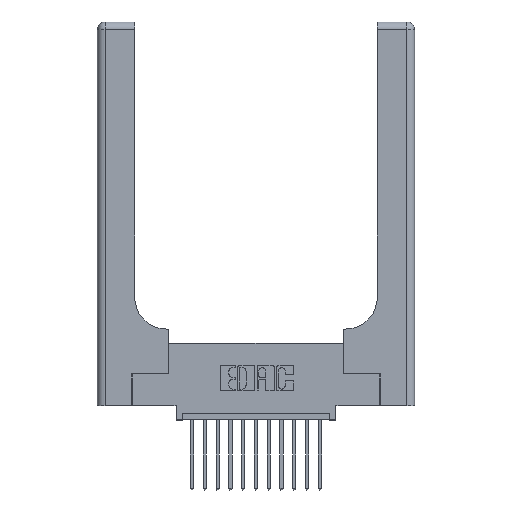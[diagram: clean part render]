
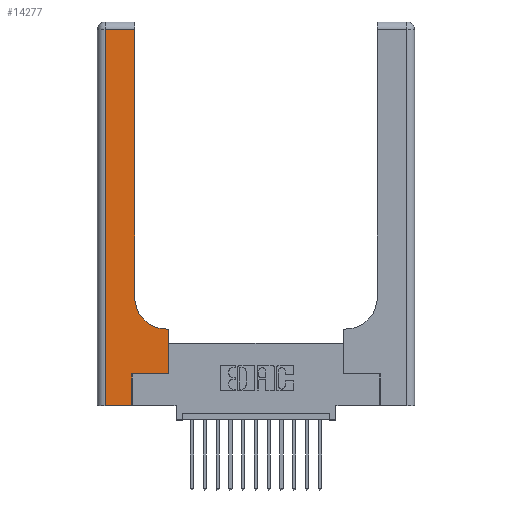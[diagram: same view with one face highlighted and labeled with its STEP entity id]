
A CAD part, top view. The second image highlights one B-rep face of the part: STEP entity #14277.
In plain terms, the highlighted planar face has unit normal (0, 0, 1).
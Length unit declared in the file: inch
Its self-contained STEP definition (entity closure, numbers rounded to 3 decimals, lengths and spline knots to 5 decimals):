
#93 = LINE ( 'NONE', #13680, #14553 ) ;
#414 = EDGE_CURVE ( 'NONE', #13971, #17429, #8022, .T. ) ;
#449 = CARTESIAN_POINT ( 'NONE',  ( 0.269, 0.25, 0.37 ) ) ;
#641 = DIRECTION ( 'NONE',  ( 0., 1., 0. ) ) ;
#719 = DIRECTION ( 'NONE',  ( -1., 0., 0. ) ) ;
#744 = VECTOR ( 'NONE', #3154, 39.37008 ) ;
#1458 = VECTOR ( 'NONE', #9864, 39.37008 ) ;
#1665 = CARTESIAN_POINT ( 'NONE',  ( 0.06, 0., 0.37 ) ) ;
#1728 = EDGE_CURVE ( 'NONE', #10482, #11210, #10958, .T. ) ;
#2546 = ORIENTED_EDGE ( 'NONE', *, *, #8735, .T. ) ;
#2795 = VECTOR ( 'NONE', #3137, 39.37008 ) ;
#2929 = CARTESIAN_POINT ( 'NONE',  ( 0.5585, 0.25, 0.37 ) ) ;
#3137 = DIRECTION ( 'NONE',  ( 1., 0., 0. ) ) ;
#3154 = DIRECTION ( 'NONE',  ( 0., 1., 0. ) ) ;
#3670 = AXIS2_PLACEMENT_3D ( 'NONE', #5417, #15176, #12306 ) ;
#4021 = EDGE_CURVE ( 'NONE', #15513, #13971, #7890, .T. ) ;
#4241 = ORIENTED_EDGE ( 'NONE', *, *, #1728, .T. ) ;
#4708 = VERTEX_POINT ( 'NONE', #8562 ) ;
#4768 = CARTESIAN_POINT ( 'NONE',  ( 0.06, 2.94, 0.37 ) ) ;
#4982 = DIRECTION ( 'NONE',  ( 0., -1., 0. ) ) ;
#5142 = VERTEX_POINT ( 'NONE', #14083 ) ;
#5417 = CARTESIAN_POINT ( 'NONE',  ( 0.5415, 0.85, 0.37 ) ) ;
#6105 = ORIENTED_EDGE ( 'NONE', *, *, #4021, .T. ) ;
#6115 = CARTESIAN_POINT ( 'NONE',  ( 0.2915, 0.6, 0.37 ) ) ;
#6341 = CARTESIAN_POINT ( 'NONE',  ( 0.2915, 2.94, 0.37 ) ) ;
#7037 = AXIS2_PLACEMENT_3D ( 'NONE', #11462, #12938, #14336 ) ;
#7217 = EDGE_CURVE ( 'NONE', #13497, #10482, #15222, .T. ) ;
#7622 = LINE ( 'NONE', #12855, #744 ) ;
#7773 = ORIENTED_EDGE ( 'NONE', *, *, #414, .T. ) ;
#7890 = LINE ( 'NONE', #17274, #14774 ) ;
#8022 = LINE ( 'NONE', #17244, #10371 ) ;
#8486 = EDGE_CURVE ( 'NONE', #9701, #4708, #16473, .T. ) ;
#8562 = CARTESIAN_POINT ( 'NONE',  ( 0.2915, 0.85, 0.37 ) ) ;
#8621 = CARTESIAN_POINT ( 'NONE',  ( 0.5585, 0.25, 0.37 ) ) ;
#8735 = EDGE_CURVE ( 'NONE', #4708, #15513, #93, .T. ) ;
#8854 = DIRECTION ( 'NONE',  ( -1., 0., 0. ) ) ;
#9108 = LINE ( 'NONE', #6115, #13655 ) ;
#9701 = VERTEX_POINT ( 'NONE', #10411 ) ;
#9825 = ORIENTED_EDGE ( 'NONE', *, *, #14733, .T. ) ;
#9864 = DIRECTION ( 'NONE',  ( 1., 0., 0. ) ) ;
#9866 = EDGE_CURVE ( 'NONE', #11210, #9701, #9108, .T. ) ;
#10101 = LINE ( 'NONE', #13857, #2795 ) ;
#10371 = VECTOR ( 'NONE', #4982, 39.37008 ) ;
#10411 = CARTESIAN_POINT ( 'NONE',  ( 0.5415, 0.6, 0.37 ) ) ;
#10482 = VERTEX_POINT ( 'NONE', #2929 ) ;
#10958 = LINE ( 'NONE', #8621, #16760 ) ;
#11210 = VERTEX_POINT ( 'NONE', #11771 ) ;
#11462 = CARTESIAN_POINT ( 'NONE',  ( 0., 3., 0.37 ) ) ;
#11725 = ORIENTED_EDGE ( 'NONE', *, *, #9866, .T. ) ;
#11771 = CARTESIAN_POINT ( 'NONE',  ( 0.5585, 0.6, 0.37 ) ) ;
#12306 = DIRECTION ( 'NONE',  ( 1., 0., 0. ) ) ;
#12855 = CARTESIAN_POINT ( 'NONE',  ( 0.269, 0., 0.37 ) ) ;
#12938 = DIRECTION ( 'NONE',  ( 0., 0., -1. ) ) ;
#13497 = VERTEX_POINT ( 'NONE', #449 ) ;
#13655 = VECTOR ( 'NONE', #8854, 39.37008 ) ;
#13680 = CARTESIAN_POINT ( 'NONE',  ( 0.2915, 3., 0.37 ) ) ;
#13857 = CARTESIAN_POINT ( 'NONE',  ( 0., 0., 0.37 ) ) ;
#13867 = EDGE_LOOP ( 'NONE', ( #2546, #6105, #7773, #17418, #9825, #16624, #4241, #11725, #16097 ) ) ;
#13971 = VERTEX_POINT ( 'NONE', #4768 ) ;
#14083 = CARTESIAN_POINT ( 'NONE',  ( 0.269, 0., 0.37 ) ) ;
#14277 = ADVANCED_FACE ( 'NONE', ( #16866 ), #15618, .F. ) ;
#14336 = DIRECTION ( 'NONE',  ( -1., 0., 0. ) ) ;
#14553 = VECTOR ( 'NONE', #16418, 39.37008 ) ;
#14733 = EDGE_CURVE ( 'NONE', #5142, #13497, #7622, .T. ) ;
#14774 = VECTOR ( 'NONE', #719, 39.37008 ) ;
#15176 = DIRECTION ( 'NONE',  ( 0., 0., -1. ) ) ;
#15222 = LINE ( 'NONE', #16728, #1458 ) ;
#15513 = VERTEX_POINT ( 'NONE', #6341 ) ;
#15618 = PLANE ( 'NONE',  #7037 ) ;
#16097 = ORIENTED_EDGE ( 'NONE', *, *, #8486, .T. ) ;
#16418 = DIRECTION ( 'NONE',  ( 0., 1., 0. ) ) ;
#16473 = CIRCLE ( 'NONE', #3670, 0.25 ) ;
#16624 = ORIENTED_EDGE ( 'NONE', *, *, #7217, .T. ) ;
#16728 = CARTESIAN_POINT ( 'NONE',  ( 0.269, 0.25, 0.37 ) ) ;
#16760 = VECTOR ( 'NONE', #641, 39.37008 ) ;
#16865 = EDGE_CURVE ( 'NONE', #17429, #5142, #10101, .T. ) ;
#16866 = FACE_OUTER_BOUND ( 'NONE', #13867, .T. ) ;
#17244 = CARTESIAN_POINT ( 'NONE',  ( 0.06, 3., 0.37 ) ) ;
#17274 = CARTESIAN_POINT ( 'NONE',  ( 0., 2.94, 0.37 ) ) ;
#17418 = ORIENTED_EDGE ( 'NONE', *, *, #16865, .T. ) ;
#17429 = VERTEX_POINT ( 'NONE', #1665 ) ;
